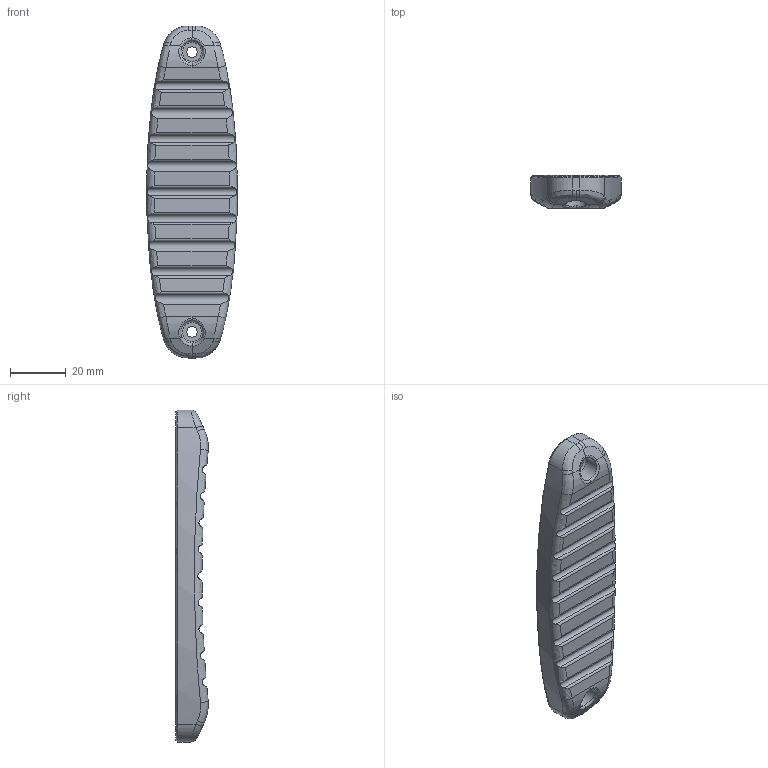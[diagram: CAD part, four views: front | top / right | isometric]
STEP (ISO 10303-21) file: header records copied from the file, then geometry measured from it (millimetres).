
FILE_DESCRIPTION(/* description */ (''),/* implementation_level */ '2;1');
FILE_NAME(/* name */ 'Buttpad.step',/* time_stamp */ '2021-10-04T06:56:30-04:00',/* author */ (''),/* organization */ (''),/* preprocessor_version */ 'ST-DEVELOPER v18.1',/* originating_system */ 'Autodesk Translation Framework v10.10.0.1391',/* authorisation */ '');
FILE_SCHEMA (('AUTOMOTIVE_DESIGN { 1 0 10303 214 3 1 1 }'));
Length unit declared in the file: millimetre
Products named in the file (1): Buttpad
Bounding box: 32.47 x 11.66 x 118.61 mm (x, y, z)
Volume: 26247.1 mm3; surface area: 9749.7 mm2
Topology: 1 solids, 1 shells, 154 faces, 376 edges, 226 vertices
Faces by surface type: bspline 68, cylinder 55, plane 15, torus 10, cone 6
Full cylindrical faces by diameter (mm): 3.8 x2, 8 x2
Entity records: 7602 total; most frequent: CARTESIAN_POINT 4437, ORIENTED_EDGE 752, DIRECTION 478, EDGE_CURVE 376, VERTEX_POINT 226, AXIS2_PLACEMENT_3D 191, B_SPLINE_CURVE_WITH_KNOTS 176, EDGE_LOOP 160
